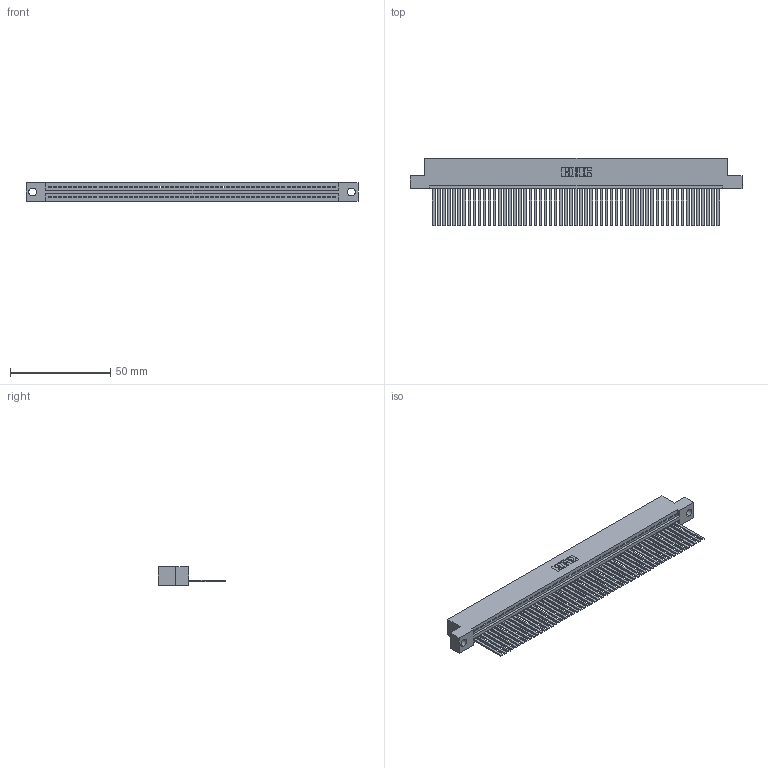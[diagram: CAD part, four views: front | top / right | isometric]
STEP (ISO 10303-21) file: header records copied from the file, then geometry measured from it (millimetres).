
FILE_DESCRIPTION (( 'STEP AP203' ), '1' );
FILE_NAME ('395-057-544-104.STEP', '2021-05-31T21:41:30', ( '' ), ( '' ), 'SwSTEP 2.0', 'SolidWorks 2020', '' );
FILE_SCHEMA (( 'CONFIG_CONTROL_DESIGN' ));
Length unit declared in the file: inch
Products named in the file (3): 345 Part_Flush Mounting Lugs - 0.156 Dia-TI; 345-292-001_345-293-144; 395-057-544-104
Assembly tree (58 placements, depth 2):
  395-057-544-104
    345 Part_Flush Mounting Lugs - 0.156 Dia-TI
    345-292-001_345-293-144  x57
Bounding box: 165.99 x 33.96 x 9.4 mm (x, y, z)
Volume: 16442.9 mm3; surface area: 23879.2 mm2
Topology: 58 solids, 58 shells, 3104 faces, 9383 edges, 6178 vertices
Faces by surface type: plane 2146, cylinder 958
Entity records: 41115 total; most frequent: CARTESIAN_POINT 7129, ORIENTED_EDGE 7118, DIRECTION 6201, EDGE_CURVE 3559, LINE 3203, VECTOR 3203, VERTEX_POINT 2370, AXIS2_PLACEMENT_3D 1499
